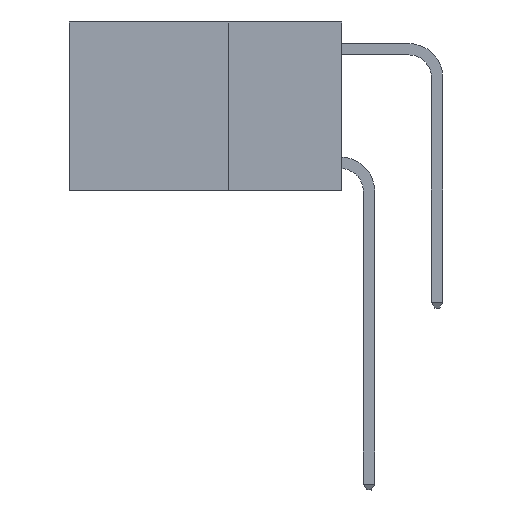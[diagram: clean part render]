
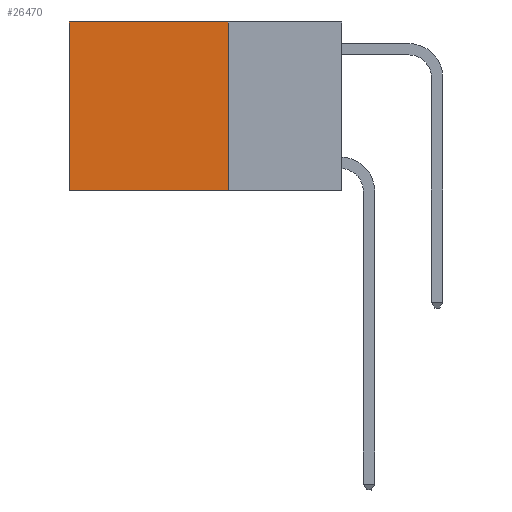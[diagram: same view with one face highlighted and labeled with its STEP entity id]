
A CAD part, left-side view. The second image highlights one B-rep face of the part: STEP entity #26470.
In plain terms, the highlighted planar face has unit normal (-1, 0, 0).
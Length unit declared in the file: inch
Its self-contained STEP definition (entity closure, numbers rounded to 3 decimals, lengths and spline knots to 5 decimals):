
#562 = DIRECTION ( 'NONE',  ( 0., 0., -1. ) ) ;
#1070 = PLANE ( 'NONE',  #24818 ) ;
#1644 = ORIENTED_EDGE ( 'NONE', *, *, #5247, .F. ) ;
#2200 = VERTEX_POINT ( 'NONE', #6697 ) ;
#2489 = VERTEX_POINT ( 'NONE', #13398 ) ;
#2571 = LINE ( 'NONE', #10715, #26231 ) ;
#3304 = DIRECTION ( 'NONE',  ( 0., 0., -1. ) ) ;
#3367 = DIRECTION ( 'NONE',  ( 0., 1., 0. ) ) ;
#4727 = DIRECTION ( 'NONE',  ( 0., 1., 0. ) ) ;
#4856 = LINE ( 'NONE', #13141, #9329 ) ;
#5108 = FACE_OUTER_BOUND ( 'NONE', #20620, .T. ) ;
#5247 = EDGE_CURVE ( 'NONE', #2200, #18065, #4856, .T. ) ;
#5316 = LINE ( 'NONE', #17822, #13115 ) ;
#5373 = DIRECTION ( 'NONE',  ( 1., 0., 0. ) ) ;
#6697 = CARTESIAN_POINT ( 'NONE',  ( 0.2625, 0.25, -0.37 ) ) ;
#9329 = VECTOR ( 'NONE', #4727, 39.37008 ) ;
#9466 = ORIENTED_EDGE ( 'NONE', *, *, #22129, .T. ) ;
#10715 = CARTESIAN_POINT ( 'NONE',  ( 0.2625, 0.25, 0. ) ) ;
#12668 = CARTESIAN_POINT ( 'NONE',  ( 0.2625, 0.6, -0.37 ) ) ;
#13115 = VECTOR ( 'NONE', #3304, 39.37008 ) ;
#13141 = CARTESIAN_POINT ( 'NONE',  ( 0.2625, 0.25, -0.37 ) ) ;
#13142 = CARTESIAN_POINT ( 'NONE',  ( 0.2625, 0.25, 0. ) ) ;
#13275 = VERTEX_POINT ( 'NONE', #22156 ) ;
#13398 = CARTESIAN_POINT ( 'NONE',  ( 0.2625, 0.25, 0. ) ) ;
#17465 = CARTESIAN_POINT ( 'NONE',  ( 0.2625, 0.25, 0. ) ) ;
#17822 = CARTESIAN_POINT ( 'NONE',  ( 0.2625, 0.6, 0. ) ) ;
#18065 = VERTEX_POINT ( 'NONE', #12668 ) ;
#19392 = LINE ( 'NONE', #13142, #25539 ) ;
#20620 = EDGE_LOOP ( 'NONE', ( #20702, #1644, #23338, #9466 ) ) ;
#20702 = ORIENTED_EDGE ( 'NONE', *, *, #23071, .T. ) ;
#21981 = EDGE_CURVE ( 'NONE', #2489, #2200, #2571, .T. ) ;
#22129 = EDGE_CURVE ( 'NONE', #2489, #13275, #19392, .T. ) ;
#22156 = CARTESIAN_POINT ( 'NONE',  ( 0.2625, 0.6, 0. ) ) ;
#23071 = EDGE_CURVE ( 'NONE', #13275, #18065, #5316, .T. ) ;
#23338 = ORIENTED_EDGE ( 'NONE', *, *, #21981, .F. ) ;
#23560 = DIRECTION ( 'NONE',  ( 0., 0., -1. ) ) ;
#24818 = AXIS2_PLACEMENT_3D ( 'NONE', #17465, #5373, #23560 ) ;
#25539 = VECTOR ( 'NONE', #3367, 39.37008 ) ;
#26231 = VECTOR ( 'NONE', #562, 39.37008 ) ;
#26470 = ADVANCED_FACE ( 'NONE', ( #5108 ), #1070, .F. ) ;
